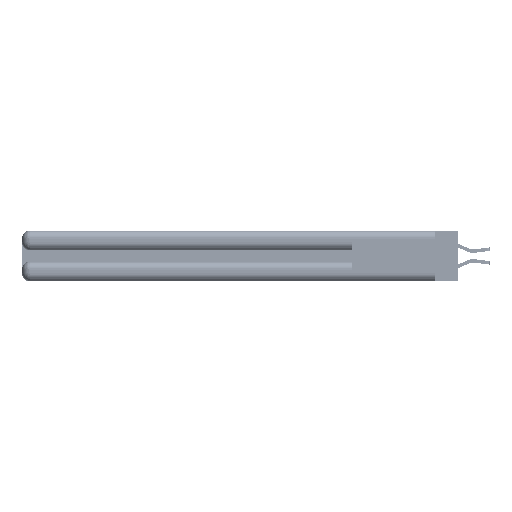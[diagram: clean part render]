
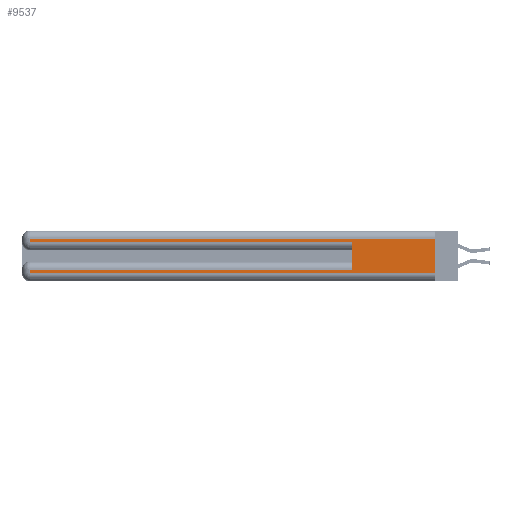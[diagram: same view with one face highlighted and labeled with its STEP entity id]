
A CAD part, left-side view. The second image highlights one B-rep face of the part: STEP entity #9537.
In plain terms, the highlighted planar face has unit normal (-1, 0, 0).
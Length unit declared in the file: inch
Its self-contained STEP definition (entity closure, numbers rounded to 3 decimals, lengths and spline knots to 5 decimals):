
#1667 = CARTESIAN_POINT ( 'NONE',  ( 0., 0., 0.31 ) ) ;
#3338 = VERTEX_POINT ( 'NONE', #39974 ) ;
#4052 = AXIS2_PLACEMENT_3D ( 'NONE', #40163, #47471, #25608 ) ;
#4294 = CARTESIAN_POINT ( 'NONE',  ( 0., 0., 0.06 ) ) ;
#4540 = CARTESIAN_POINT ( 'NONE',  ( 0., 2.94, 0.285 ) ) ;
#4723 = DIRECTION ( 'NONE',  ( 0., -1., 0. ) ) ;
#5609 = ORIENTED_EDGE ( 'NONE', *, *, #6136, .T. ) ;
#6136 = EDGE_CURVE ( 'NONE', #12555, #3338, #24275, .T. ) ;
#6983 = LINE ( 'NONE', #12643, #25546 ) ;
#7093 = LINE ( 'NONE', #18349, #35412 ) ;
#7263 = CARTESIAN_POINT ( 'NONE',  ( 0., 2.94, 0.37 ) ) ;
#7352 = VECTOR ( 'NONE', #9585, 39.37008 ) ;
#8929 = VECTOR ( 'NONE', #22809, 39.37008 ) ;
#9149 = EDGE_CURVE ( 'NONE', #35355, #16488, #47410, .T. ) ;
#9537 = ADVANCED_FACE ( 'NONE', ( #46230 ), #21886, .F. ) ;
#9562 = EDGE_CURVE ( 'NONE', #36753, #22788, #7093, .T. ) ;
#9585 = DIRECTION ( 'NONE',  ( 0., 0., -1. ) ) ;
#10827 = ORIENTED_EDGE ( 'NONE', *, *, #9562, .T. ) ;
#11024 = DIRECTION ( 'NONE',  ( 0., 0., -1. ) ) ;
#11828 = ORIENTED_EDGE ( 'NONE', *, *, #19281, .T. ) ;
#12298 = EDGE_CURVE ( 'NONE', #12555, #16488, #29978, .T. ) ;
#12472 = ORIENTED_EDGE ( 'NONE', *, *, #12298, .F. ) ;
#12555 = VERTEX_POINT ( 'NONE', #21225 ) ;
#12643 = CARTESIAN_POINT ( 'NONE',  ( 0., 0., 0.37 ) ) ;
#12705 = EDGE_CURVE ( 'NONE', #22788, #35355, #31082, .T. ) ;
#14697 = VECTOR ( 'NONE', #4723, 39.37008 ) ;
#15628 = CARTESIAN_POINT ( 'NONE',  ( 0., 0., 0.285 ) ) ;
#15662 = ORIENTED_EDGE ( 'NONE', *, *, #12705, .T. ) ;
#16429 = DIRECTION ( 'NONE',  ( 0., 0., -1. ) ) ;
#16488 = VERTEX_POINT ( 'NONE', #38427 ) ;
#17264 = LINE ( 'NONE', #24318, #7352 ) ;
#18349 = CARTESIAN_POINT ( 'NONE',  ( 0., 0., 0.31 ) ) ;
#19281 = EDGE_CURVE ( 'NONE', #3338, #36951, #17264, .T. ) ;
#19798 = CARTESIAN_POINT ( 'NONE',  ( 0., 0.6, 0.145 ) ) ;
#21225 = CARTESIAN_POINT ( 'NONE',  ( 0., 0.6, 0.085 ) ) ;
#21292 = CARTESIAN_POINT ( 'NONE',  ( 0., 2.94, 0.06 ) ) ;
#21886 = PLANE ( 'NONE',  #4052 ) ;
#22043 = DIRECTION ( 'NONE',  ( 0., 1., 0. ) ) ;
#22282 = EDGE_LOOP ( 'NONE', ( #34127, #10827, #15662, #29470, #12472, #5609, #11828, #42769 ) ) ;
#22788 = VERTEX_POINT ( 'NONE', #25656 ) ;
#22809 = DIRECTION ( 'NONE',  ( 0., -1., 0. ) ) ;
#23098 = VECTOR ( 'NONE', #35085, 39.37008 ) ;
#23878 = CARTESIAN_POINT ( 'NONE',  ( 0., 0., 0.06 ) ) ;
#24275 = LINE ( 'NONE', #38756, #23098 ) ;
#24318 = CARTESIAN_POINT ( 'NONE',  ( 0., 2.94, 0.37 ) ) ;
#25546 = VECTOR ( 'NONE', #16429, 39.37008 ) ;
#25608 = DIRECTION ( 'NONE',  ( 0., 0., -1. ) ) ;
#25656 = CARTESIAN_POINT ( 'NONE',  ( 0., 2.94, 0.31 ) ) ;
#29470 = ORIENTED_EDGE ( 'NONE', *, *, #9149, .T. ) ;
#29978 = LINE ( 'NONE', #19798, #38527 ) ;
#31082 = LINE ( 'NONE', #7263, #39622 ) ;
#34127 = ORIENTED_EDGE ( 'NONE', *, *, #46699, .F. ) ;
#35085 = DIRECTION ( 'NONE',  ( 0., 1., 0. ) ) ;
#35355 = VERTEX_POINT ( 'NONE', #4540 ) ;
#35412 = VECTOR ( 'NONE', #22043, 39.37008 ) ;
#36753 = VERTEX_POINT ( 'NONE', #1667 ) ;
#36951 = VERTEX_POINT ( 'NONE', #21292 ) ;
#37383 = VERTEX_POINT ( 'NONE', #23878 ) ;
#38269 = DIRECTION ( 'NONE',  ( 0., 0., 1. ) ) ;
#38318 = LINE ( 'NONE', #4294, #8929 ) ;
#38427 = CARTESIAN_POINT ( 'NONE',  ( 0., 0.6, 0.285 ) ) ;
#38527 = VECTOR ( 'NONE', #38269, 39.37008 ) ;
#38756 = CARTESIAN_POINT ( 'NONE',  ( 0., 0., 0.085 ) ) ;
#39622 = VECTOR ( 'NONE', #11024, 39.37008 ) ;
#39974 = CARTESIAN_POINT ( 'NONE',  ( 0., 2.94, 0.085 ) ) ;
#40163 = CARTESIAN_POINT ( 'NONE',  ( 0., 0., 0.37 ) ) ;
#40315 = EDGE_CURVE ( 'NONE', #36951, #37383, #38318, .T. ) ;
#42769 = ORIENTED_EDGE ( 'NONE', *, *, #40315, .T. ) ;
#46230 = FACE_OUTER_BOUND ( 'NONE', #22282, .T. ) ;
#46699 = EDGE_CURVE ( 'NONE', #36753, #37383, #6983, .T. ) ;
#47410 = LINE ( 'NONE', #15628, #14697 ) ;
#47471 = DIRECTION ( 'NONE',  ( 1., 0., 0. ) ) ;
